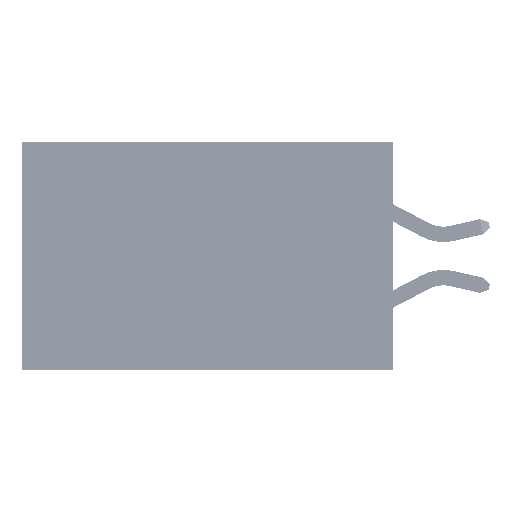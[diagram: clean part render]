
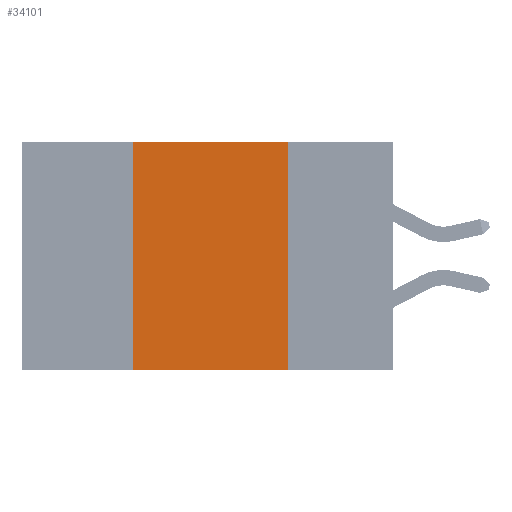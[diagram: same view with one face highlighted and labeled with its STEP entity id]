
A CAD part, left-side view. The second image highlights one B-rep face of the part: STEP entity #34101.
In plain terms, the highlighted planar face has unit normal (-1, 0, 0).
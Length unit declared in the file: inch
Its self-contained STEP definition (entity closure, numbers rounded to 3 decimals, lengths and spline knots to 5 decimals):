
#539 = VERTEX_POINT ( 'NONE', #12446 ) ;
#970 = CARTESIAN_POINT ( 'NONE',  ( 0., 0.17, 0. ) ) ;
#1576 = ORIENTED_EDGE ( 'NONE', *, *, #45968, .F. ) ;
#5184 = CARTESIAN_POINT ( 'NONE',  ( 0., 0.42, 0. ) ) ;
#6811 = EDGE_CURVE ( 'NONE', #27493, #24351, #24904, .T. ) ;
#7412 = VERTEX_POINT ( 'NONE', #28600 ) ;
#10259 = FACE_OUTER_BOUND ( 'NONE', #43373, .T. ) ;
#11026 = DIRECTION ( 'NONE',  ( 0., 0., -1. ) ) ;
#11609 = DIRECTION ( 'NONE',  ( 0., -1., 0. ) ) ;
#11693 = ORIENTED_EDGE ( 'NONE', *, *, #38818, .F. ) ;
#12446 = CARTESIAN_POINT ( 'NONE',  ( 0., 0.17, -0.37 ) ) ;
#14930 = AXIS2_PLACEMENT_3D ( 'NONE', #34781, #19376, #11026 ) ;
#19376 = DIRECTION ( 'NONE',  ( 1., 0., 0. ) ) ;
#21012 = DIRECTION ( 'NONE',  ( 0., 0., 1. ) ) ;
#24351 = VERTEX_POINT ( 'NONE', #25768 ) ;
#24904 = LINE ( 'NONE', #5184, #39157 ) ;
#25127 = DIRECTION ( 'NONE',  ( 0., 0., -1. ) ) ;
#25768 = CARTESIAN_POINT ( 'NONE',  ( 0., 0.42, 0. ) ) ;
#26255 = VECTOR ( 'NONE', #25127, 39.37008 ) ;
#27493 = VERTEX_POINT ( 'NONE', #47827 ) ;
#28600 = CARTESIAN_POINT ( 'NONE',  ( 0., 0.17, 0. ) ) ;
#29494 = ORIENTED_EDGE ( 'NONE', *, *, #6811, .F. ) ;
#30816 = LINE ( 'NONE', #970, #26255 ) ;
#31323 = PLANE ( 'NONE',  #14930 ) ;
#31561 = LINE ( 'NONE', #48460, #38339 ) ;
#33861 = ORIENTED_EDGE ( 'NONE', *, *, #40041, .T. ) ;
#34101 = ADVANCED_FACE ( 'NONE', ( #10259 ), #31323, .F. ) ;
#34781 = CARTESIAN_POINT ( 'NONE',  ( 0., 0.6, 0. ) ) ;
#35700 = CARTESIAN_POINT ( 'NONE',  ( 0., 0.6, -0.37 ) ) ;
#36318 = DIRECTION ( 'NONE',  ( 0., -1., 0. ) ) ;
#38028 = LINE ( 'NONE', #35700, #47332 ) ;
#38339 = VECTOR ( 'NONE', #36318, 39.37008 ) ;
#38818 = EDGE_CURVE ( 'NONE', #24351, #7412, #31561, .T. ) ;
#39157 = VECTOR ( 'NONE', #21012, 39.37008 ) ;
#40041 = EDGE_CURVE ( 'NONE', #27493, #539, #38028, .T. ) ;
#43373 = EDGE_LOOP ( 'NONE', ( #1576, #11693, #29494, #33861 ) ) ;
#45968 = EDGE_CURVE ( 'NONE', #7412, #539, #30816, .T. ) ;
#47332 = VECTOR ( 'NONE', #11609, 39.37008 ) ;
#47827 = CARTESIAN_POINT ( 'NONE',  ( 0., 0.42, -0.37 ) ) ;
#48460 = CARTESIAN_POINT ( 'NONE',  ( 0., 0.6, 0. ) ) ;
